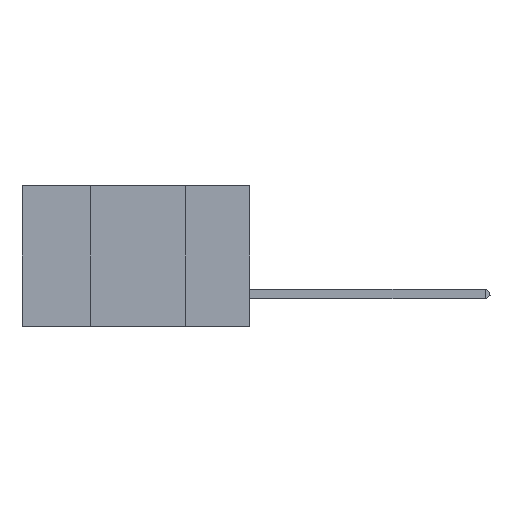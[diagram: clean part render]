
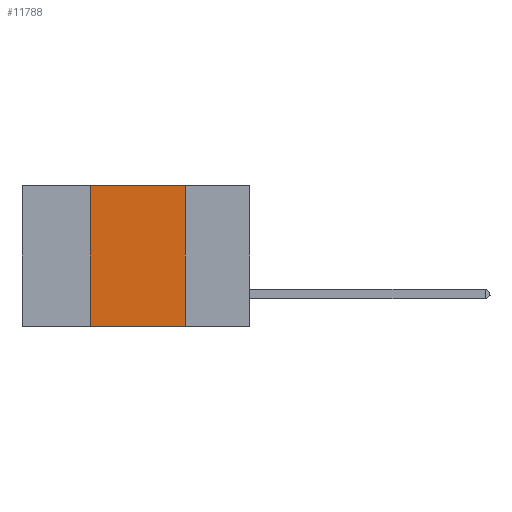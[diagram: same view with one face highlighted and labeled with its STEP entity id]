
A CAD part, left-side view. The second image highlights one B-rep face of the part: STEP entity #11788.
In plain terms, the highlighted planar face has unit normal (-1, 0, 0).
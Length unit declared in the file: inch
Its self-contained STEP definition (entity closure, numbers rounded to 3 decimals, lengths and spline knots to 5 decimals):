
#199 = CARTESIAN_POINT ( 'NONE',  ( 0., 0.42, 0. ) ) ;
#1058 = VECTOR ( 'NONE', #19306, 39.37008 ) ;
#2788 = DIRECTION ( 'NONE',  ( 0., -1., 0. ) ) ;
#4353 = DIRECTION ( 'NONE',  ( 0., 0., -1. ) ) ;
#4678 = VECTOR ( 'NONE', #26598, 39.37008 ) ;
#5067 = EDGE_CURVE ( 'NONE', #22291, #20908, #19750, .T. ) ;
#5144 = VERTEX_POINT ( 'NONE', #199 ) ;
#6312 = VERTEX_POINT ( 'NONE', #9357 ) ;
#6423 = CARTESIAN_POINT ( 'NONE',  ( 0., 0.42, 0. ) ) ;
#8633 = LINE ( 'NONE', #6423, #4678 ) ;
#8889 = CARTESIAN_POINT ( 'NONE',  ( 0., 0.17, 0. ) ) ;
#9010 = EDGE_LOOP ( 'NONE', ( #12426, #22584, #19491, #16456 ) ) ;
#9357 = CARTESIAN_POINT ( 'NONE',  ( 0., 0.17, 0. ) ) ;
#9645 = FACE_OUTER_BOUND ( 'NONE', #9010, .T. ) ;
#10504 = CARTESIAN_POINT ( 'NONE',  ( 0., 0.42, -0.37 ) ) ;
#10932 = CARTESIAN_POINT ( 'NONE',  ( 0., 0.6, -0.37 ) ) ;
#11788 = ADVANCED_FACE ( 'NONE', ( #9645 ), #21405, .F. ) ;
#11990 = EDGE_CURVE ( 'NONE', #6312, #20908, #29081, .T. ) ;
#12426 = ORIENTED_EDGE ( 'NONE', *, *, #11990, .F. ) ;
#14214 = DIRECTION ( 'NONE',  ( 0., 0., -1. ) ) ;
#16177 = LINE ( 'NONE', #27524, #16400 ) ;
#16400 = VECTOR ( 'NONE', #2788, 39.37008 ) ;
#16456 = ORIENTED_EDGE ( 'NONE', *, *, #5067, .T. ) ;
#16551 = EDGE_CURVE ( 'NONE', #5144, #6312, #16177, .T. ) ;
#18615 = CARTESIAN_POINT ( 'NONE',  ( 0., 0.6, 0. ) ) ;
#19306 = DIRECTION ( 'NONE',  ( 0., -1., 0. ) ) ;
#19491 = ORIENTED_EDGE ( 'NONE', *, *, #28672, .F. ) ;
#19750 = LINE ( 'NONE', #10932, #1058 ) ;
#20908 = VERTEX_POINT ( 'NONE', #26076 ) ;
#21405 = PLANE ( 'NONE',  #28742 ) ;
#22291 = VERTEX_POINT ( 'NONE', #10504 ) ;
#22584 = ORIENTED_EDGE ( 'NONE', *, *, #16551, .F. ) ;
#25398 = DIRECTION ( 'NONE',  ( 1., 0., 0. ) ) ;
#25422 = VECTOR ( 'NONE', #4353, 39.37008 ) ;
#26076 = CARTESIAN_POINT ( 'NONE',  ( 0., 0.17, -0.37 ) ) ;
#26598 = DIRECTION ( 'NONE',  ( 0., 0., 1. ) ) ;
#27524 = CARTESIAN_POINT ( 'NONE',  ( 0., 0.6, 0. ) ) ;
#28672 = EDGE_CURVE ( 'NONE', #22291, #5144, #8633, .T. ) ;
#28742 = AXIS2_PLACEMENT_3D ( 'NONE', #18615, #25398, #14214 ) ;
#29081 = LINE ( 'NONE', #8889, #25422 ) ;
